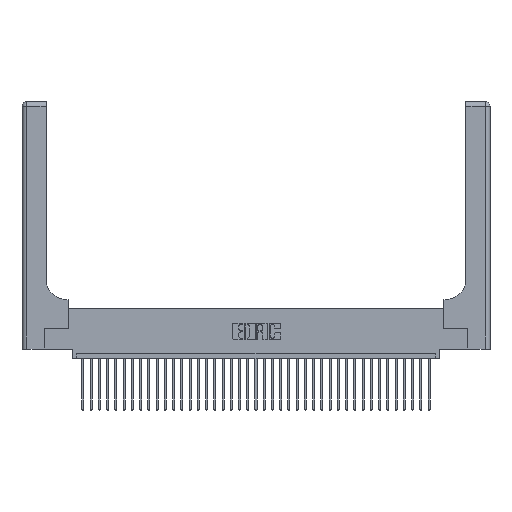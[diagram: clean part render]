
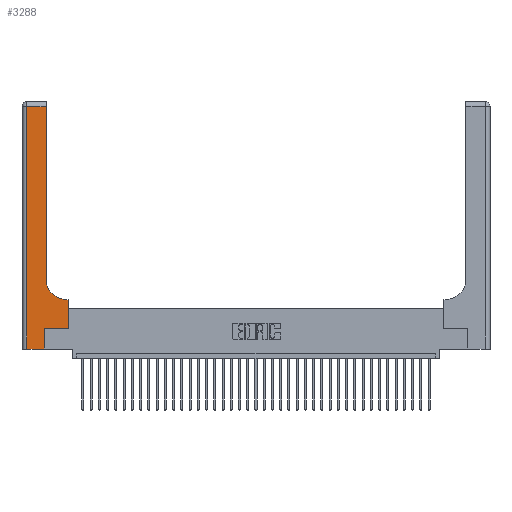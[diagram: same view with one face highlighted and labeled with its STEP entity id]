
A CAD part, top view. The second image highlights one B-rep face of the part: STEP entity #3288.
In plain terms, the highlighted planar face has unit normal (0, 0, 1).
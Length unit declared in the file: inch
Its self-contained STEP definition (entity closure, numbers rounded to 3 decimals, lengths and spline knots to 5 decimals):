
#541 = EDGE_CURVE ( 'NONE', #9371, #22798, #2732, .T. ) ;
#563 = CARTESIAN_POINT ( 'NONE',  ( 0., 0., 0.37 ) ) ;
#2229 = CARTESIAN_POINT ( 'NONE',  ( 0.2915, 0.85, 0.37 ) ) ;
#2732 = LINE ( 'NONE', #9830, #20802 ) ;
#3288 = ADVANCED_FACE ( 'NONE', ( #20595 ), #8349, .F. ) ;
#3402 = ORIENTED_EDGE ( 'NONE', *, *, #25272, .T. ) ;
#3503 = VECTOR ( 'NONE', #14298, 39.37008 ) ;
#3815 = VECTOR ( 'NONE', #26627, 39.37008 ) ;
#4422 = DIRECTION ( 'NONE',  ( -1., 0., 0. ) ) ;
#4489 = LINE ( 'NONE', #5151, #34420 ) ;
#5132 = CARTESIAN_POINT ( 'NONE',  ( 0.5415, 0.6, 0.37 ) ) ;
#5151 = CARTESIAN_POINT ( 'NONE',  ( 0.06, 3., 0.37 ) ) ;
#5329 = CARTESIAN_POINT ( 'NONE',  ( 0., 3., 0.37 ) ) ;
#6152 = EDGE_CURVE ( 'NONE', #29306, #24987, #21941, .T. ) ;
#6777 = VERTEX_POINT ( 'NONE', #24856 ) ;
#6872 = DIRECTION ( 'NONE',  ( 0., 0., -1. ) ) ;
#8106 = LINE ( 'NONE', #15491, #18971 ) ;
#8349 = PLANE ( 'NONE',  #36062 ) ;
#9371 = VERTEX_POINT ( 'NONE', #18664 ) ;
#9437 = DIRECTION ( 'NONE',  ( 0., 1., 0. ) ) ;
#9501 = VERTEX_POINT ( 'NONE', #2229 ) ;
#9618 = ORIENTED_EDGE ( 'NONE', *, *, #541, .T. ) ;
#9830 = CARTESIAN_POINT ( 'NONE',  ( 0.2915, 0.6, 0.37 ) ) ;
#10048 = EDGE_CURVE ( 'NONE', #6777, #19618, #8106, .T. ) ;
#10055 = DIRECTION ( 'NONE',  ( -1., 0., 0. ) ) ;
#10417 = DIRECTION ( 'NONE',  ( 0., -1., 0. ) ) ;
#10482 = EDGE_CURVE ( 'NONE', #22798, #9501, #13508, .T. ) ;
#10840 = VERTEX_POINT ( 'NONE', #25166 ) ;
#10961 = ORIENTED_EDGE ( 'NONE', *, *, #10482, .T. ) ;
#11142 = DIRECTION ( 'NONE',  ( -1., 0., 0. ) ) ;
#13212 = VERTEX_POINT ( 'NONE', #18399 ) ;
#13237 = ORIENTED_EDGE ( 'NONE', *, *, #6152, .T. ) ;
#13296 = CARTESIAN_POINT ( 'NONE',  ( 0.269, 0., 0.37 ) ) ;
#13508 = CIRCLE ( 'NONE', #26160, 0.25 ) ;
#13650 = VECTOR ( 'NONE', #36287, 39.37008 ) ;
#14244 = LINE ( 'NONE', #17107, #23725 ) ;
#14298 = DIRECTION ( 'NONE',  ( 1., 0., 0. ) ) ;
#15491 = CARTESIAN_POINT ( 'NONE',  ( 0., 2.94, 0.37 ) ) ;
#17107 = CARTESIAN_POINT ( 'NONE',  ( 0.5585, 0.25, 0.37 ) ) ;
#17224 = DIRECTION ( 'NONE',  ( 0., 1., 0. ) ) ;
#17951 = ORIENTED_EDGE ( 'NONE', *, *, #31358, .T. ) ;
#18399 = CARTESIAN_POINT ( 'NONE',  ( 0.5585, 0.25, 0.37 ) ) ;
#18664 = CARTESIAN_POINT ( 'NONE',  ( 0.5585, 0.6, 0.37 ) ) ;
#18971 = VECTOR ( 'NONE', #10055, 39.37008 ) ;
#19075 = LINE ( 'NONE', #29433, #19989 ) ;
#19351 = CARTESIAN_POINT ( 'NONE',  ( 0.06, 0., 0.37 ) ) ;
#19618 = VERTEX_POINT ( 'NONE', #19924 ) ;
#19851 = LINE ( 'NONE', #23019, #3503 ) ;
#19924 = CARTESIAN_POINT ( 'NONE',  ( 0.06, 2.94, 0.37 ) ) ;
#19989 = VECTOR ( 'NONE', #9437, 39.37008 ) ;
#20595 = FACE_OUTER_BOUND ( 'NONE', #30890, .T. ) ;
#20802 = VECTOR ( 'NONE', #4422, 39.37008 ) ;
#21203 = ORIENTED_EDGE ( 'NONE', *, *, #22074, .T. ) ;
#21941 = LINE ( 'NONE', #563, #3815 ) ;
#22074 = EDGE_CURVE ( 'NONE', #13212, #9371, #14244, .T. ) ;
#22798 = VERTEX_POINT ( 'NONE', #5132 ) ;
#23019 = CARTESIAN_POINT ( 'NONE',  ( 0.269, 0.25, 0.37 ) ) ;
#23168 = LINE ( 'NONE', #13296, #13650 ) ;
#23725 = VECTOR ( 'NONE', #17224, 39.37008 ) ;
#23880 = EDGE_CURVE ( 'NONE', #24987, #10840, #23168, .T. ) ;
#24856 = CARTESIAN_POINT ( 'NONE',  ( 0.2915, 2.94, 0.37 ) ) ;
#24987 = VERTEX_POINT ( 'NONE', #27020 ) ;
#25166 = CARTESIAN_POINT ( 'NONE',  ( 0.269, 0.25, 0.37 ) ) ;
#25272 = EDGE_CURVE ( 'NONE', #19618, #29306, #4489, .T. ) ;
#26160 = AXIS2_PLACEMENT_3D ( 'NONE', #30160, #6872, #27510 ) ;
#26627 = DIRECTION ( 'NONE',  ( 1., 0., 0. ) ) ;
#27020 = CARTESIAN_POINT ( 'NONE',  ( 0.269, 0., 0.37 ) ) ;
#27510 = DIRECTION ( 'NONE',  ( 1., 0., 0. ) ) ;
#27654 = ORIENTED_EDGE ( 'NONE', *, *, #23880, .T. ) ;
#28498 = DIRECTION ( 'NONE',  ( 0., 0., -1. ) ) ;
#29166 = ORIENTED_EDGE ( 'NONE', *, *, #10048, .T. ) ;
#29306 = VERTEX_POINT ( 'NONE', #19351 ) ;
#29433 = CARTESIAN_POINT ( 'NONE',  ( 0.2915, 3., 0.37 ) ) ;
#30160 = CARTESIAN_POINT ( 'NONE',  ( 0.5415, 0.85, 0.37 ) ) ;
#30890 = EDGE_LOOP ( 'NONE', ( #17951, #29166, #3402, #13237, #27654, #36991, #21203, #9618, #10961 ) ) ;
#31358 = EDGE_CURVE ( 'NONE', #9501, #6777, #19075, .T. ) ;
#32837 = EDGE_CURVE ( 'NONE', #10840, #13212, #19851, .T. ) ;
#34420 = VECTOR ( 'NONE', #10417, 39.37008 ) ;
#36062 = AXIS2_PLACEMENT_3D ( 'NONE', #5329, #28498, #11142 ) ;
#36287 = DIRECTION ( 'NONE',  ( 0., 1., 0. ) ) ;
#36991 = ORIENTED_EDGE ( 'NONE', *, *, #32837, .T. ) ;
